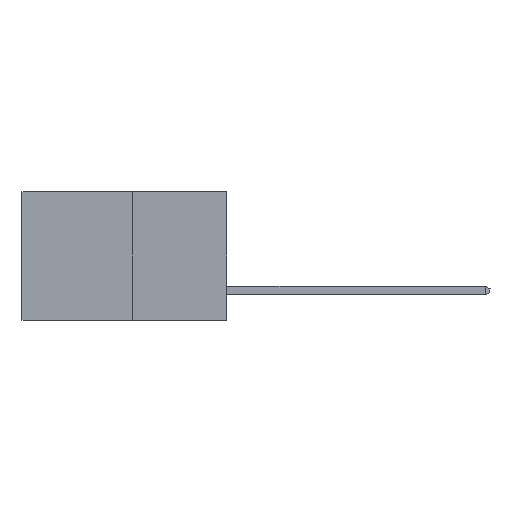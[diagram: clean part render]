
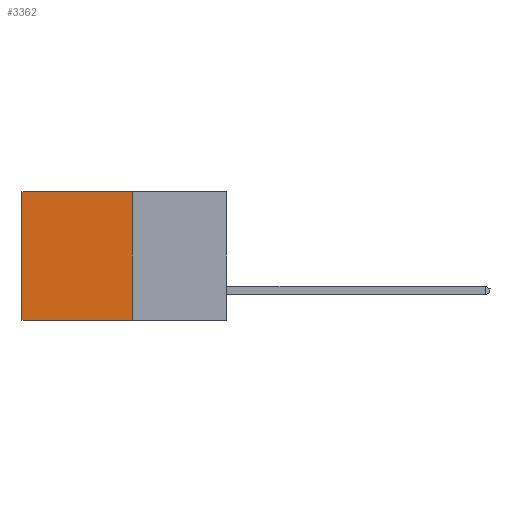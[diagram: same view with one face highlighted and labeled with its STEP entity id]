
A CAD part, left-side view. The second image highlights one B-rep face of the part: STEP entity #3362.
In plain terms, the highlighted planar face has unit normal (-1, 0, 0).
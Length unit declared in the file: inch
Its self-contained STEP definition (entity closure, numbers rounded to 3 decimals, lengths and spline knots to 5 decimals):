
#253 = CARTESIAN_POINT ( 'NONE',  ( 0.277, 0.59, -0.37 ) ) ;
#879 = AXIS2_PLACEMENT_3D ( 'NONE', #3878, #4402, #2955 ) ;
#882 = LINE ( 'NONE', #4062, #4982 ) ;
#956 = VERTEX_POINT ( 'NONE', #7366 ) ;
#1213 = EDGE_LOOP ( 'NONE', ( #5838, #1512, #1468, #1637 ) ) ;
#1372 = FACE_OUTER_BOUND ( 'NONE', #1213, .T. ) ;
#1443 = EDGE_CURVE ( 'NONE', #2475, #2364, #4430, .T. ) ;
#1468 = ORIENTED_EDGE ( 'NONE', *, *, #2734, .F. ) ;
#1512 = ORIENTED_EDGE ( 'NONE', *, *, #1443, .F. ) ;
#1637 = ORIENTED_EDGE ( 'NONE', *, *, #3645, .T. ) ;
#1647 = DIRECTION ( 'NONE',  ( 0., 0., -1. ) ) ;
#1935 = DIRECTION ( 'NONE',  ( 0., 1., 0. ) ) ;
#2364 = VERTEX_POINT ( 'NONE', #253 ) ;
#2475 = VERTEX_POINT ( 'NONE', #3413 ) ;
#2516 = VECTOR ( 'NONE', #4074, 39.37008 ) ;
#2651 = CARTESIAN_POINT ( 'NONE',  ( 0.277, 0.27, -0.37 ) ) ;
#2734 = EDGE_CURVE ( 'NONE', #956, #2475, #7838, .T. ) ;
#2955 = DIRECTION ( 'NONE',  ( 0., 0., -1. ) ) ;
#3362 = ADVANCED_FACE ( 'NONE', ( #1372 ), #3667, .F. ) ;
#3413 = CARTESIAN_POINT ( 'NONE',  ( 0.277, 0.27, -0.37 ) ) ;
#3645 = EDGE_CURVE ( 'NONE', #956, #7575, #882, .T. ) ;
#3667 = PLANE ( 'NONE',  #879 ) ;
#3878 = CARTESIAN_POINT ( 'NONE',  ( 0.277, 0.27, -0.37 ) ) ;
#3992 = DIRECTION ( 'NONE',  ( 0., 1., 0. ) ) ;
#4062 = CARTESIAN_POINT ( 'NONE',  ( 0.277, 0.27, 0. ) ) ;
#4074 = DIRECTION ( 'NONE',  ( 0., 0., -1. ) ) ;
#4175 = EDGE_CURVE ( 'NONE', #7575, #2364, #4303, .T. ) ;
#4303 = LINE ( 'NONE', #8693, #7585 ) ;
#4402 = DIRECTION ( 'NONE',  ( 1., 0., 0. ) ) ;
#4430 = LINE ( 'NONE', #6888, #6011 ) ;
#4982 = VECTOR ( 'NONE', #3992, 39.37008 ) ;
#5321 = CARTESIAN_POINT ( 'NONE',  ( 0.277, 0.59, 0. ) ) ;
#5838 = ORIENTED_EDGE ( 'NONE', *, *, #4175, .T. ) ;
#6011 = VECTOR ( 'NONE', #1935, 39.37008 ) ;
#6888 = CARTESIAN_POINT ( 'NONE',  ( 0.277, 0.27, -0.37 ) ) ;
#7366 = CARTESIAN_POINT ( 'NONE',  ( 0.277, 0.27, 0. ) ) ;
#7575 = VERTEX_POINT ( 'NONE', #5321 ) ;
#7585 = VECTOR ( 'NONE', #1647, 39.37008 ) ;
#7838 = LINE ( 'NONE', #2651, #2516 ) ;
#8693 = CARTESIAN_POINT ( 'NONE',  ( 0.277, 0.59, -0.37 ) ) ;
